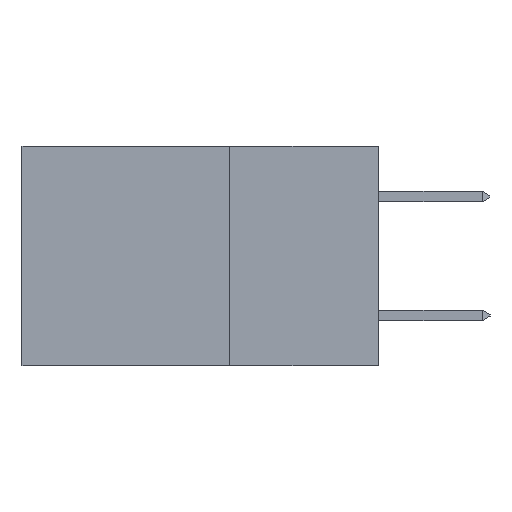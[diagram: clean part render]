
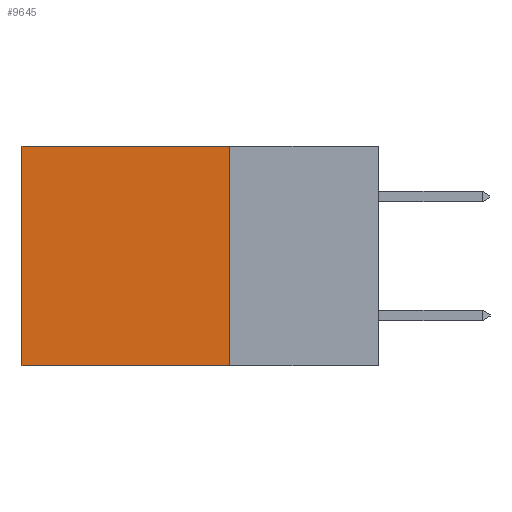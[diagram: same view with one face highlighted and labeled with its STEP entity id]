
A CAD part, left-side view. The second image highlights one B-rep face of the part: STEP entity #9645.
In plain terms, the highlighted planar face has unit normal (-1, 0, 0).
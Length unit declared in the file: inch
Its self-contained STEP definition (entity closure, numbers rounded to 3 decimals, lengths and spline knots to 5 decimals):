
#536 = VERTEX_POINT ( 'NONE', #4976 ) ;
#823 = FACE_OUTER_BOUND ( 'NONE', #2346, .T. ) ;
#1488 = VECTOR ( 'NONE', #7597, 39.37008 ) ;
#1555 = DIRECTION ( 'NONE',  ( 1., 0., 0. ) ) ;
#1632 = LINE ( 'NONE', #9418, #9386 ) ;
#1917 = VERTEX_POINT ( 'NONE', #4719 ) ;
#2206 = VERTEX_POINT ( 'NONE', #7309 ) ;
#2287 = ORIENTED_EDGE ( 'NONE', *, *, #4312, .T. ) ;
#2346 = EDGE_LOOP ( 'NONE', ( #2287, #3038, #5561, #2968 ) ) ;
#2968 = ORIENTED_EDGE ( 'NONE', *, *, #6324, .T. ) ;
#3038 = ORIENTED_EDGE ( 'NONE', *, *, #8803, .F. ) ;
#3085 = VECTOR ( 'NONE', #8681, 39.37008 ) ;
#3346 = CARTESIAN_POINT ( 'NONE',  ( 0.2615, 0.25, -0.37 ) ) ;
#3673 = CARTESIAN_POINT ( 'NONE',  ( 0.2615, 0.25, 0. ) ) ;
#4047 = CARTESIAN_POINT ( 'NONE',  ( 0.2615, 0.25, -0.37 ) ) ;
#4095 = EDGE_CURVE ( 'NONE', #1917, #4865, #5249, .T. ) ;
#4208 = LINE ( 'NONE', #3673, #6261 ) ;
#4312 = EDGE_CURVE ( 'NONE', #536, #2206, #7452, .T. ) ;
#4719 = CARTESIAN_POINT ( 'NONE',  ( 0.2615, 0.25, 0. ) ) ;
#4865 = VERTEX_POINT ( 'NONE', #3346 ) ;
#4976 = CARTESIAN_POINT ( 'NONE',  ( 0.2615, 0.6, 0. ) ) ;
#5249 = LINE ( 'NONE', #8791, #3085 ) ;
#5561 = ORIENTED_EDGE ( 'NONE', *, *, #4095, .F. ) ;
#6261 = VECTOR ( 'NONE', #8047, 39.37008 ) ;
#6324 = EDGE_CURVE ( 'NONE', #1917, #536, #4208, .T. ) ;
#6364 = PLANE ( 'NONE',  #8828 ) ;
#7039 = DIRECTION ( 'NONE',  ( 0., 0., -1. ) ) ;
#7309 = CARTESIAN_POINT ( 'NONE',  ( 0.2615, 0.6, -0.37 ) ) ;
#7452 = LINE ( 'NONE', #7625, #1488 ) ;
#7597 = DIRECTION ( 'NONE',  ( 0., 0., -1. ) ) ;
#7625 = CARTESIAN_POINT ( 'NONE',  ( 0.2615, 0.6, -0.37 ) ) ;
#8047 = DIRECTION ( 'NONE',  ( 0., 1., 0. ) ) ;
#8080 = DIRECTION ( 'NONE',  ( 0., 1., 0. ) ) ;
#8681 = DIRECTION ( 'NONE',  ( 0., 0., -1. ) ) ;
#8791 = CARTESIAN_POINT ( 'NONE',  ( 0.2615, 0.25, -0.37 ) ) ;
#8803 = EDGE_CURVE ( 'NONE', #4865, #2206, #1632, .T. ) ;
#8828 = AXIS2_PLACEMENT_3D ( 'NONE', #4047, #1555, #7039 ) ;
#9386 = VECTOR ( 'NONE', #8080, 39.37008 ) ;
#9418 = CARTESIAN_POINT ( 'NONE',  ( 0.2615, 0.25, -0.37 ) ) ;
#9645 = ADVANCED_FACE ( 'NONE', ( #823 ), #6364, .F. ) ;
